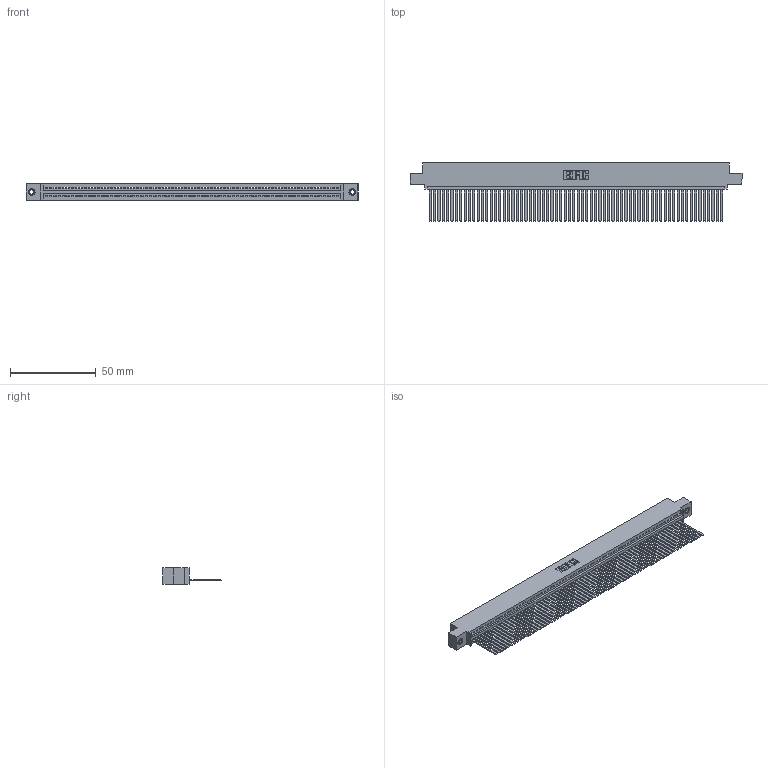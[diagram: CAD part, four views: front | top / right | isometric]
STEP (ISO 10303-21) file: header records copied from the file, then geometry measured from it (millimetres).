
FILE_DESCRIPTION (( 'STEP AP203' ), '1' );
FILE_NAME ('395-068-544-407.STEP', '2019-10-25T18:40:49', ( '' ), ( '' ), 'SwSTEP 2.0', 'SolidWorks 2016', '' );
FILE_SCHEMA (( 'CONFIG_CONTROL_DESIGN' ));
Length unit declared in the file: inch
Products named in the file (4): 345-292-001_345-293-144; 395-068-544-407; 345-250-001_345-250-005-103; 345 Part_0.110 Offset - 0.156 Dia-TI
Assembly tree (71 placements, depth 2):
  395-068-544-407
    345 Part_0.110 Offset - 0.156 Dia-TI
    345-292-001_345-293-144  x68
    345-250-001_345-250-005-103  x2
Bounding box: 193.93 x 33.96 x 9.4 mm (x, y, z)
Volume: 19333.2 mm3; surface area: 28524.1 mm2
Topology: 71 solids, 71 shells, 3726 faces, 11233 edges, 7390 vertices
Faces by surface type: plane 2564, cylinder 1146, cone 12, torus 4
Entity records: 48812 total; most frequent: CARTESIAN_POINT 8435, ORIENTED_EDGE 8430, DIRECTION 7353, EDGE_CURVE 4215, LINE 3795, VECTOR 3795, VERTEX_POINT 2804, AXIS2_PLACEMENT_3D 1779
